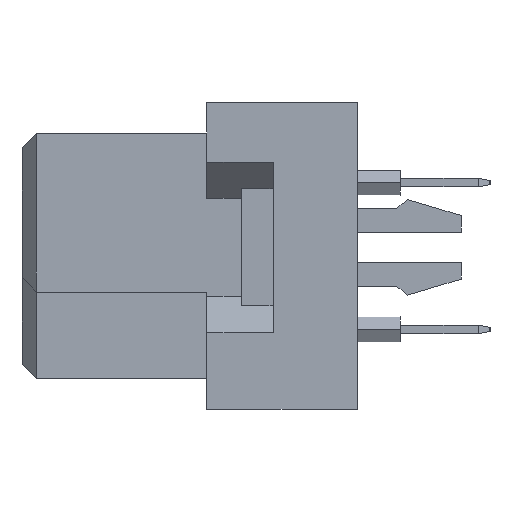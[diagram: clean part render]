
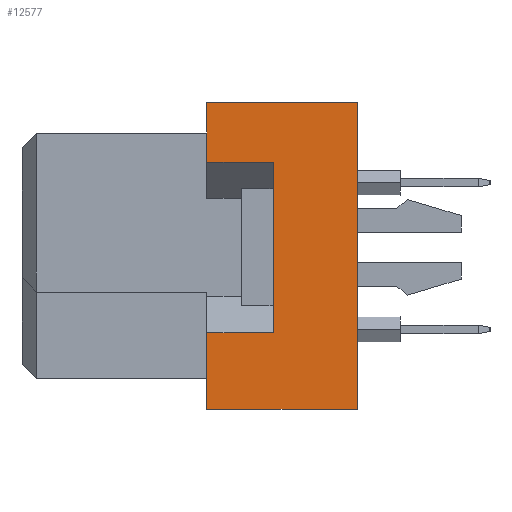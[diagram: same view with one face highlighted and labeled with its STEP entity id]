
A CAD part, left-side view. The second image highlights one B-rep face of the part: STEP entity #12577.
In plain terms, the highlighted planar face has unit normal (-1, 0, 0).
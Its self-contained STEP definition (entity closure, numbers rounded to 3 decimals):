
#666 = VERTEX_POINT ( 'NONE', #27261 ) ;
#1103 = LINE ( 'NONE', #22551, #24253 ) ;
#1571 = LINE ( 'NONE', #31472, #29283 ) ;
#3235 = DIRECTION ( 'NONE',  ( 0., 1., 0. ) ) ;
#3424 = VECTOR ( 'NONE', #34309, 1000. ) ;
#3920 = LINE ( 'NONE', #13152, #22817 ) ;
#4308 = DIRECTION ( 'NONE',  ( 0., 0., 1. ) ) ;
#5080 = ORIENTED_EDGE ( 'NONE', *, *, #27607, .F. ) ;
#5193 = VECTOR ( 'NONE', #17120, 1000. ) ;
#6091 = VERTEX_POINT ( 'NONE', #7918 ) ;
#6201 = ORIENTED_EDGE ( 'NONE', *, *, #18271, .F. ) ;
#6377 = PLANE ( 'NONE',  #27014 ) ;
#6978 = VERTEX_POINT ( 'NONE', #37861 ) ;
#7225 = LINE ( 'NONE', #28690, #3424 ) ;
#7918 = CARTESIAN_POINT ( 'NONE',  ( -47.5, -6.4, 3.25 ) ) ;
#9384 = FACE_OUTER_BOUND ( 'NONE', #24069, .T. ) ;
#9534 = CARTESIAN_POINT ( 'NONE',  ( -47.5, -8.7, -2.65 ) ) ;
#9651 = LINE ( 'NONE', #36529, #9815 ) ;
#9815 = VECTOR ( 'NONE', #3235, 1000. ) ;
#11221 = VERTEX_POINT ( 'NONE', #11752 ) ;
#11609 = EDGE_CURVE ( 'NONE', #6091, #15139, #26551, .T. ) ;
#11752 = CARTESIAN_POINT ( 'NONE',  ( -47.5, -8.7, 3.25 ) ) ;
#11807 = CARTESIAN_POINT ( 'NONE',  ( -47.5, -11.6, 5.3 ) ) ;
#12577 = ADVANCED_FACE ( 'NONE', ( #9384 ), #6377, .T. ) ;
#12650 = EDGE_CURVE ( 'NONE', #666, #15139, #36462, .T. ) ;
#13152 = CARTESIAN_POINT ( 'NONE',  ( -47.5, -11.6, 5.3 ) ) ;
#14699 = CARTESIAN_POINT ( 'NONE',  ( -47.5, -6.4, -2.65 ) ) ;
#15139 = VERTEX_POINT ( 'NONE', #21841 ) ;
#15154 = ORIENTED_EDGE ( 'NONE', *, *, #11609, .F. ) ;
#15341 = LINE ( 'NONE', #22128, #37415 ) ;
#16730 = ORIENTED_EDGE ( 'NONE', *, *, #12650, .T. ) ;
#16750 = VECTOR ( 'NONE', #24047, 1000. ) ;
#17120 = DIRECTION ( 'NONE',  ( 0., 0., 1. ) ) ;
#17254 = VERTEX_POINT ( 'NONE', #9534 ) ;
#18271 = EDGE_CURVE ( 'NONE', #17254, #11221, #1103, .T. ) ;
#19526 = ORIENTED_EDGE ( 'NONE', *, *, #30499, .T. ) ;
#21841 = CARTESIAN_POINT ( 'NONE',  ( -47.5, -6.4, 5.3 ) ) ;
#22128 = CARTESIAN_POINT ( 'NONE',  ( -47.5, -6.4, -5.3 ) ) ;
#22442 = DIRECTION ( 'NONE',  ( 0., 1., 0. ) ) ;
#22551 = CARTESIAN_POINT ( 'NONE',  ( -47.5, -8.7, -2.65 ) ) ;
#22817 = VECTOR ( 'NONE', #31219, 1000. ) ;
#24047 = DIRECTION ( 'NONE',  ( 0., 1., 0. ) ) ;
#24069 = EDGE_LOOP ( 'NONE', ( #37215, #37540, #5080, #19526, #16730, #15154, #31808, #6201 ) ) ;
#24166 = VERTEX_POINT ( 'NONE', #32935 ) ;
#24253 = VECTOR ( 'NONE', #4308, 1000. ) ;
#26551 = LINE ( 'NONE', #29964, #5193 ) ;
#26855 = DIRECTION ( 'NONE',  ( -1., 0., 0. ) ) ;
#27014 = AXIS2_PLACEMENT_3D ( 'NONE', #36845, #26855, #27455 ) ;
#27049 = EDGE_CURVE ( 'NONE', #24166, #27323, #15341, .T. ) ;
#27261 = CARTESIAN_POINT ( 'NONE',  ( -47.5, -11.6, 5.3 ) ) ;
#27323 = VERTEX_POINT ( 'NONE', #14699 ) ;
#27455 = DIRECTION ( 'NONE',  ( 0., 0., 1. ) ) ;
#27504 = EDGE_CURVE ( 'NONE', #11221, #6091, #9651, .T. ) ;
#27607 = EDGE_CURVE ( 'NONE', #6978, #24166, #7225, .T. ) ;
#28690 = CARTESIAN_POINT ( 'NONE',  ( -47.5, -11.6, -5.3 ) ) ;
#29283 = VECTOR ( 'NONE', #22442, 1000. ) ;
#29964 = CARTESIAN_POINT ( 'NONE',  ( -47.5, -6.4, -5.3 ) ) ;
#30499 = EDGE_CURVE ( 'NONE', #6978, #666, #3920, .T. ) ;
#31219 = DIRECTION ( 'NONE',  ( 0., 0., 1. ) ) ;
#31472 = CARTESIAN_POINT ( 'NONE',  ( -47.5, -8.7, -2.65 ) ) ;
#31808 = ORIENTED_EDGE ( 'NONE', *, *, #27504, .F. ) ;
#32935 = CARTESIAN_POINT ( 'NONE',  ( -47.5, -6.4, -5.3 ) ) ;
#34309 = DIRECTION ( 'NONE',  ( 0., 1., 0. ) ) ;
#36462 = LINE ( 'NONE', #11807, #16750 ) ;
#36529 = CARTESIAN_POINT ( 'NONE',  ( -47.5, -8.7, 3.25 ) ) ;
#36845 = CARTESIAN_POINT ( 'NONE',  ( -47.5, -11.6, 5.3 ) ) ;
#37215 = ORIENTED_EDGE ( 'NONE', *, *, #37431, .T. ) ;
#37415 = VECTOR ( 'NONE', #39586, 1000. ) ;
#37431 = EDGE_CURVE ( 'NONE', #17254, #27323, #1571, .T. ) ;
#37540 = ORIENTED_EDGE ( 'NONE', *, *, #27049, .F. ) ;
#37861 = CARTESIAN_POINT ( 'NONE',  ( -47.5, -11.6, -5.3 ) ) ;
#39586 = DIRECTION ( 'NONE',  ( 0., 0., 1. ) ) ;
